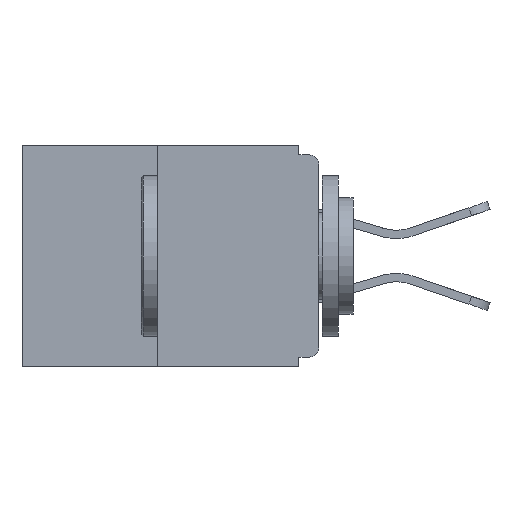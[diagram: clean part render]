
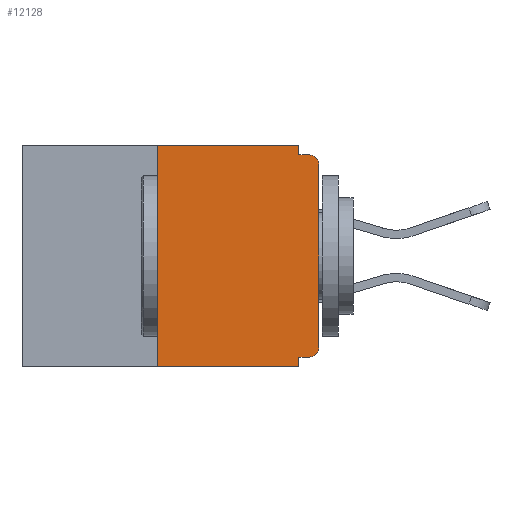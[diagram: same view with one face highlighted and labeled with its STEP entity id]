
A CAD part, left-side view. The second image highlights one B-rep face of the part: STEP entity #12128.
In plain terms, the highlighted planar face has unit normal (-1, 0, 0).
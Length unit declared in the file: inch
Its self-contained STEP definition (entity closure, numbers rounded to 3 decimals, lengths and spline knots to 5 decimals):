
#359 = ORIENTED_EDGE ( 'NONE', *, *, #14168, .T. ) ;
#918 = LINE ( 'NONE', #12461, #5912 ) ;
#1294 = VERTEX_POINT ( 'NONE', #5371 ) ;
#1314 = CIRCLE ( 'NONE', #11868, 0.015 ) ;
#2439 = FACE_OUTER_BOUND ( 'NONE', #22324, .T. ) ;
#2512 = CARTESIAN_POINT ( 'NONE',  ( 0., 0.031, -0.343 ) ) ;
#2742 = DIRECTION ( 'NONE',  ( 0., 0., -1. ) ) ;
#2835 = CARTESIAN_POINT ( 'NONE',  ( 0., 0.031, -0.328 ) ) ;
#2918 = CARTESIAN_POINT ( 'NONE',  ( 0., 0.25, -0.343 ) ) ;
#3235 = LINE ( 'NONE', #6382, #25579 ) ;
#3341 = LINE ( 'NONE', #2512, #25356 ) ;
#3372 = VERTEX_POINT ( 'NONE', #15363 ) ;
#3665 = ORIENTED_EDGE ( 'NONE', *, *, #12298, .F. ) ;
#3926 = PLANE ( 'NONE',  #7828 ) ;
#4597 = CIRCLE ( 'NONE', #21646, 0.015 ) ;
#4898 = DIRECTION ( 'NONE',  ( -1., 0., 0. ) ) ;
#5008 = ORIENTED_EDGE ( 'NONE', *, *, #8953, .F. ) ;
#5026 = DIRECTION ( 'NONE',  ( 0., 0., -1. ) ) ;
#5204 = ORIENTED_EDGE ( 'NONE', *, *, #6027, .F. ) ;
#5371 = CARTESIAN_POINT ( 'NONE',  ( 0., 0., -0.03 ) ) ;
#5798 = DIRECTION ( 'NONE',  ( 1., 0., 0. ) ) ;
#5912 = VECTOR ( 'NONE', #6446, 39.37008 ) ;
#5996 = VERTEX_POINT ( 'NONE', #2835 ) ;
#6027 = EDGE_CURVE ( 'NONE', #6464, #23601, #14248, .T. ) ;
#6320 = CARTESIAN_POINT ( 'NONE',  ( 0., 0.25, 0. ) ) ;
#6372 = VECTOR ( 'NONE', #22017, 39.37008 ) ;
#6382 = CARTESIAN_POINT ( 'NONE',  ( 0., 0.25, 0. ) ) ;
#6446 = DIRECTION ( 'NONE',  ( 0., -1., 0. ) ) ;
#6464 = VERTEX_POINT ( 'NONE', #6320 ) ;
#6866 = EDGE_CURVE ( 'NONE', #3372, #24727, #1314, .T. ) ;
#7053 = VERTEX_POINT ( 'NONE', #19245 ) ;
#7164 = VECTOR ( 'NONE', #17083, 39.37008 ) ;
#7675 = CARTESIAN_POINT ( 'NONE',  ( 0., 0.031, -0.343 ) ) ;
#7742 = CARTESIAN_POINT ( 'NONE',  ( 0., 0.46, 0. ) ) ;
#7828 = AXIS2_PLACEMENT_3D ( 'NONE', #7742, #5798, #21879 ) ;
#8049 = CARTESIAN_POINT ( 'NONE',  ( 0., 0., -0.328 ) ) ;
#8600 = ORIENTED_EDGE ( 'NONE', *, *, #6866, .T. ) ;
#8601 = LINE ( 'NONE', #10669, #25554 ) ;
#8674 = EDGE_CURVE ( 'NONE', #24727, #1294, #8601, .T. ) ;
#8953 = EDGE_CURVE ( 'NONE', #3372, #5996, #19222, .T. ) ;
#10669 = CARTESIAN_POINT ( 'NONE',  ( 0., 0., 0. ) ) ;
#10799 = DIRECTION ( 'NONE',  ( 0., 0., -1. ) ) ;
#11424 = CARTESIAN_POINT ( 'NONE',  ( 0., 0., -0.015 ) ) ;
#11427 = ORIENTED_EDGE ( 'NONE', *, *, #17555, .F. ) ;
#11491 = CARTESIAN_POINT ( 'NONE',  ( 0., 0.031, -0.015 ) ) ;
#11868 = AXIS2_PLACEMENT_3D ( 'NONE', #25270, #21597, #19373 ) ;
#12128 = ADVANCED_FACE ( 'NONE', ( #2439 ), #3926, .F. ) ;
#12298 = EDGE_CURVE ( 'NONE', #5996, #24790, #3341, .T. ) ;
#12461 = CARTESIAN_POINT ( 'NONE',  ( 0., 0.46, -0.343 ) ) ;
#12482 = DIRECTION ( 'NONE',  ( 0., 0., 1. ) ) ;
#12981 = EDGE_CURVE ( 'NONE', #1294, #7053, #4597, .T. ) ;
#13581 = CARTESIAN_POINT ( 'NONE',  ( 0., 0., -0.313 ) ) ;
#14168 = EDGE_CURVE ( 'NONE', #22365, #24790, #918, .T. ) ;
#14248 = LINE ( 'NONE', #18709, #18623 ) ;
#14945 = CARTESIAN_POINT ( 'NONE',  ( 0., 0.015, -0.03 ) ) ;
#15363 = CARTESIAN_POINT ( 'NONE',  ( 0., 0.015, -0.328 ) ) ;
#17083 = DIRECTION ( 'NONE',  ( 0., -1., 0. ) ) ;
#17390 = EDGE_CURVE ( 'NONE', #22365, #6464, #3235, .T. ) ;
#17555 = EDGE_CURVE ( 'NONE', #23601, #24661, #18339, .T. ) ;
#18339 = LINE ( 'NONE', #20868, #23689 ) ;
#18436 = ORIENTED_EDGE ( 'NONE', *, *, #8674, .T. ) ;
#18623 = VECTOR ( 'NONE', #22933, 39.37008 ) ;
#18709 = CARTESIAN_POINT ( 'NONE',  ( 0., 0.46, 0. ) ) ;
#19222 = LINE ( 'NONE', #8049, #6372 ) ;
#19245 = CARTESIAN_POINT ( 'NONE',  ( 0., 0.015, -0.015 ) ) ;
#19373 = DIRECTION ( 'NONE',  ( 0., 0., -1. ) ) ;
#19831 = ORIENTED_EDGE ( 'NONE', *, *, #17390, .F. ) ;
#20868 = CARTESIAN_POINT ( 'NONE',  ( 0., 0.031, 0. ) ) ;
#21597 = DIRECTION ( 'NONE',  ( -1., 0., 0. ) ) ;
#21646 = AXIS2_PLACEMENT_3D ( 'NONE', #14945, #4898, #2742 ) ;
#21839 = ORIENTED_EDGE ( 'NONE', *, *, #12981, .T. ) ;
#21879 = DIRECTION ( 'NONE',  ( 0., 0., -1. ) ) ;
#22017 = DIRECTION ( 'NONE',  ( 0., 1., 0. ) ) ;
#22108 = ORIENTED_EDGE ( 'NONE', *, *, #25865, .F. ) ;
#22324 = EDGE_LOOP ( 'NONE', ( #5204, #19831, #359, #3665, #5008, #8600, #18436, #21839, #22108, #11427 ) ) ;
#22365 = VERTEX_POINT ( 'NONE', #2918 ) ;
#22933 = DIRECTION ( 'NONE',  ( 0., -1., 0. ) ) ;
#23601 = VERTEX_POINT ( 'NONE', #24758 ) ;
#23689 = VECTOR ( 'NONE', #5026, 39.37008 ) ;
#24661 = VERTEX_POINT ( 'NONE', #11491 ) ;
#24688 = DIRECTION ( 'NONE',  ( 0., 0., 1. ) ) ;
#24727 = VERTEX_POINT ( 'NONE', #13581 ) ;
#24758 = CARTESIAN_POINT ( 'NONE',  ( 0., 0.031, 0. ) ) ;
#24790 = VERTEX_POINT ( 'NONE', #7675 ) ;
#24807 = LINE ( 'NONE', #11424, #7164 ) ;
#25270 = CARTESIAN_POINT ( 'NONE',  ( 0., 0.015, -0.313 ) ) ;
#25356 = VECTOR ( 'NONE', #10799, 39.37008 ) ;
#25554 = VECTOR ( 'NONE', #24688, 39.37008 ) ;
#25579 = VECTOR ( 'NONE', #12482, 39.37008 ) ;
#25865 = EDGE_CURVE ( 'NONE', #24661, #7053, #24807, .T. ) ;
